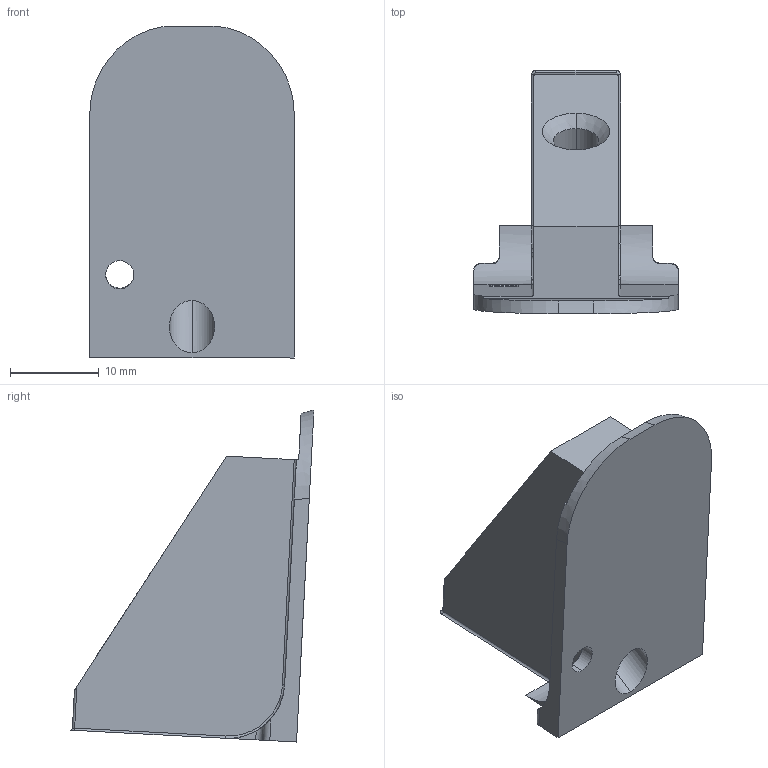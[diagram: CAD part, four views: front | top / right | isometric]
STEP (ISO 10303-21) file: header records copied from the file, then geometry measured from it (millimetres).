
FILE_DESCRIPTION (( 'STEP AP214' ), '1' );
FILE_NAME ('6.STEP', '2013-09-29T07:10:01', ( 'elpi' ), ( '' ), 'SwSTEP 2.0', 'SolidWorks 2013', '' );
FILE_SCHEMA (( 'AUTOMOTIVE_DESIGN' ));
Length unit declared in the file: millimetre
Products named in the file (1): 6
Bounding box: 23.02 x 27.48 x 37.41 mm (x, y, z)
Volume: 6070.2 mm3; surface area: 3638.8 mm2
Topology: 1 solids, 1 shells, 45 faces, 119 edges, 76 vertices
Faces by surface type: cylinder 19, plane 16, torus 6, cone 4
Entity records: 1755 total; most frequent: CARTESIAN_POINT 606, ORIENTED_EDGE 238, DIRECTION 229, EDGE_CURVE 119, AXIS2_PLACEMENT_3D 85, VERTEX_POINT 76, VECTOR 59, LINE 59
